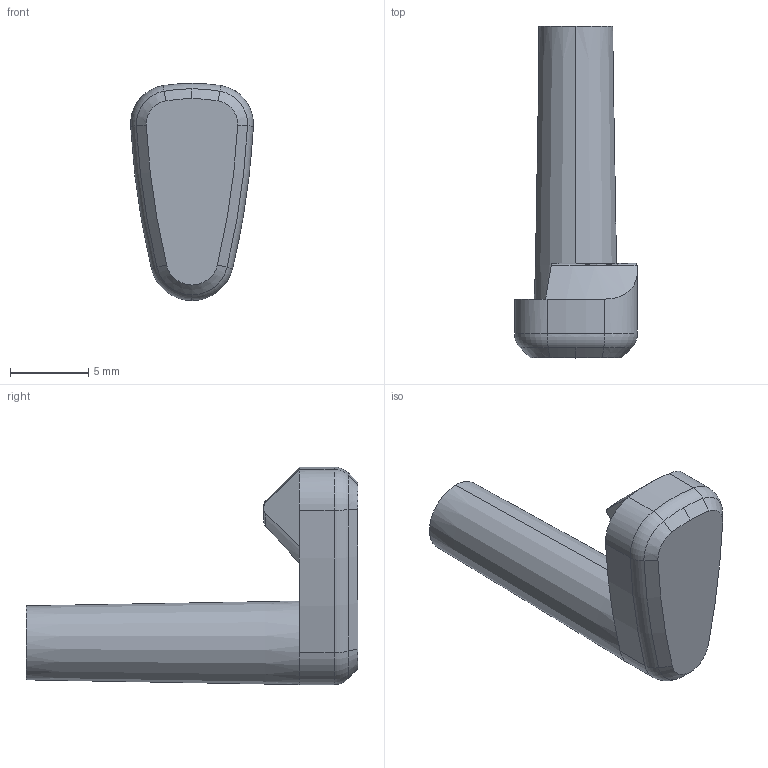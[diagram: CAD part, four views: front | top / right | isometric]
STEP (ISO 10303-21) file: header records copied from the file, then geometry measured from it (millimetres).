
FILE_DESCRIPTION (( 'STEP AP214' ), '1' );
FILE_NAME ('Barrel_Lock.step', '2015-01-13T04:29:59', ( '' ), ( '' ), 'SwSTEP 2.0', 'SolidWorks 2015', '' );
FILE_SCHEMA (( 'AUTOMOTIVE_DESIGN' ));
Length unit declared in the file: millimetre
Products named in the file (1): Barrel_Lock
Bounding box: 7.85 x 21.25 x 13.91 mm (x, y, z)
Volume: 696.8 mm3; surface area: 584.8 mm2
Topology: 1 solids, 1 shells, 31 faces, 71 edges, 42 vertices
Faces by surface type: cone 12, torus 8, cylinder 7, plane 4
Entity records: 935 total; most frequent: DIRECTION 175, CARTESIAN_POINT 174, ORIENTED_EDGE 142, AXIS2_PLACEMENT_3D 77, EDGE_CURVE 71, CIRCLE 45, VERTEX_POINT 42, ADVANCED_FACE 31
